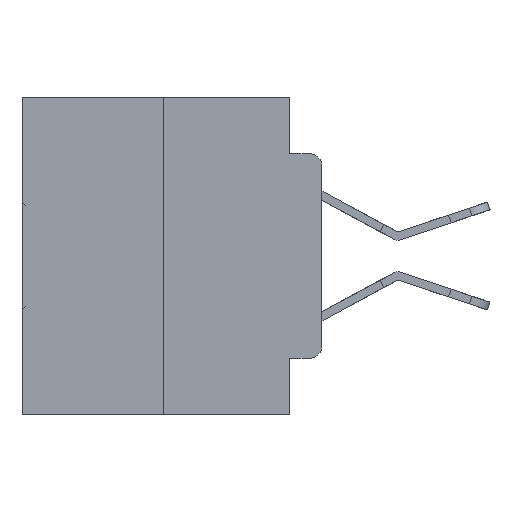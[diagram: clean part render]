
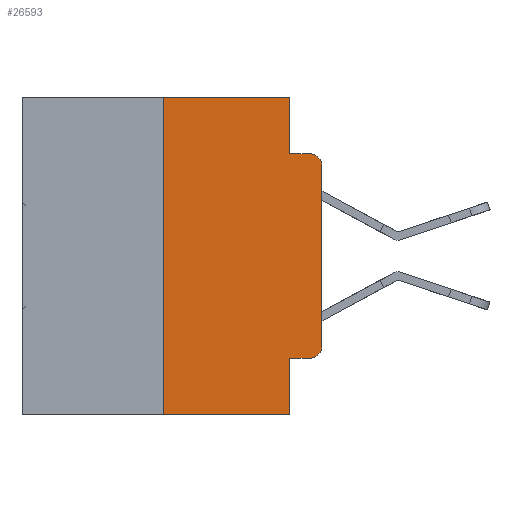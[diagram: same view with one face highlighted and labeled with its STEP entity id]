
A CAD part, left-side view. The second image highlights one B-rep face of the part: STEP entity #26593.
In plain terms, the highlighted planar face has unit normal (-1, 0, 0).
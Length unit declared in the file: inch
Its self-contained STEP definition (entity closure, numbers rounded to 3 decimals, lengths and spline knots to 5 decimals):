
#27 = CARTESIAN_POINT ( 'NONE',  ( 0., 0.051, -0.0885 ) ) ;
#431 = DIRECTION ( 'NONE',  ( 0., -1., 0. ) ) ;
#745 = CARTESIAN_POINT ( 'NONE',  ( 0., 0.051, -0.4115 ) ) ;
#867 = AXIS2_PLACEMENT_3D ( 'NONE', #20750, #5692, #33012 ) ;
#901 = LINE ( 'NONE', #29747, #17784 ) ;
#994 = VERTEX_POINT ( 'NONE', #6682 ) ;
#1021 = EDGE_CURVE ( 'NONE', #27551, #27570, #901, .T. ) ;
#2595 = LINE ( 'NONE', #27, #9815 ) ;
#2596 = ORIENTED_EDGE ( 'NONE', *, *, #13693, .T. ) ;
#2701 = ORIENTED_EDGE ( 'NONE', *, *, #3934, .T. ) ;
#2768 = VERTEX_POINT ( 'NONE', #18240 ) ;
#2932 = ORIENTED_EDGE ( 'NONE', *, *, #31230, .F. ) ;
#2973 = DIRECTION ( 'NONE',  ( 0., -1., 0. ) ) ;
#3149 = FACE_OUTER_BOUND ( 'NONE', #29541, .T. ) ;
#3934 = EDGE_CURVE ( 'NONE', #27551, #26898, #23631, .T. ) ;
#4164 = CARTESIAN_POINT ( 'NONE',  ( 0., 0., -0.1085 ) ) ;
#5619 = CARTESIAN_POINT ( 'NONE',  ( 0., 0.25, 0. ) ) ;
#5692 = DIRECTION ( 'NONE',  ( 1., 0., 0. ) ) ;
#5788 = CARTESIAN_POINT ( 'NONE',  ( 0., 0.25, -0.5 ) ) ;
#6343 = DIRECTION ( 'NONE',  ( 0., 0., 1. ) ) ;
#6682 = CARTESIAN_POINT ( 'NONE',  ( 0., 0.02, -0.4115 ) ) ;
#7279 = VECTOR ( 'NONE', #13715, 39.37008 ) ;
#7805 = CARTESIAN_POINT ( 'NONE',  ( 0., 0., 0. ) ) ;
#8265 = LINE ( 'NONE', #26204, #10832 ) ;
#8440 = ORIENTED_EDGE ( 'NONE', *, *, #26118, .T. ) ;
#8484 = VECTOR ( 'NONE', #28814, 39.37008 ) ;
#8527 = CIRCLE ( 'NONE', #26545, 0.02 ) ;
#8709 = EDGE_CURVE ( 'NONE', #27570, #29041, #8265, .T. ) ;
#9815 = VECTOR ( 'NONE', #20842, 39.37008 ) ;
#10832 = VECTOR ( 'NONE', #431, 39.37008 ) ;
#10989 = CARTESIAN_POINT ( 'NONE',  ( 0., 0.051, 0. ) ) ;
#11209 = EDGE_CURVE ( 'NONE', #16443, #33388, #2595, .T. ) ;
#12436 = CARTESIAN_POINT ( 'NONE',  ( 0., 0.051, 0. ) ) ;
#13693 = EDGE_CURVE ( 'NONE', #16097, #994, #21564, .T. ) ;
#13715 = DIRECTION ( 'NONE',  ( 0., -1., 0. ) ) ;
#14390 = CARTESIAN_POINT ( 'NONE',  ( 0., 0.051, -0.5 ) ) ;
#14406 = CIRCLE ( 'NONE', #29677, 0.02 ) ;
#14635 = ORIENTED_EDGE ( 'NONE', *, *, #11209, .F. ) ;
#15655 = DIRECTION ( 'NONE',  ( -1., 0., 0. ) ) ;
#15794 = DIRECTION ( 'NONE',  ( 0., 0., -1. ) ) ;
#16097 = VERTEX_POINT ( 'NONE', #25193 ) ;
#16354 = CARTESIAN_POINT ( 'NONE',  ( 0., 0.051, 0. ) ) ;
#16443 = VERTEX_POINT ( 'NONE', #16570 ) ;
#16570 = CARTESIAN_POINT ( 'NONE',  ( 0., 0.051, -0.0885 ) ) ;
#17191 = DIRECTION ( 'NONE',  ( -1., 0., 0. ) ) ;
#17784 = VECTOR ( 'NONE', #6343, 39.37008 ) ;
#18180 = LINE ( 'NONE', #12436, #32018 ) ;
#18240 = CARTESIAN_POINT ( 'NONE',  ( 0., 0., -0.3915 ) ) ;
#18380 = CARTESIAN_POINT ( 'NONE',  ( 0., 0.02, -0.3915 ) ) ;
#19927 = CARTESIAN_POINT ( 'NONE',  ( 0., 0.02, -0.1085 ) ) ;
#20366 = VECTOR ( 'NONE', #15794, 39.37008 ) ;
#20750 = CARTESIAN_POINT ( 'NONE',  ( 0., 0.473, 0. ) ) ;
#20842 = DIRECTION ( 'NONE',  ( 0., -1., 0. ) ) ;
#21564 = LINE ( 'NONE', #745, #7279 ) ;
#23044 = VECTOR ( 'NONE', #2973, 39.37008 ) ;
#23481 = PLANE ( 'NONE',  #867 ) ;
#23488 = DIRECTION ( 'NONE',  ( 0., 0., -1. ) ) ;
#23491 = LINE ( 'NONE', #10989, #20366 ) ;
#23631 = LINE ( 'NONE', #28598, #23044 ) ;
#23675 = DIRECTION ( 'NONE',  ( 0., 0., -1. ) ) ;
#24698 = EDGE_CURVE ( 'NONE', #994, #2768, #14406, .T. ) ;
#25193 = CARTESIAN_POINT ( 'NONE',  ( 0., 0.051, -0.4115 ) ) ;
#25556 = ORIENTED_EDGE ( 'NONE', *, *, #1021, .F. ) ;
#26118 = EDGE_CURVE ( 'NONE', #2768, #31346, #26241, .T. ) ;
#26204 = CARTESIAN_POINT ( 'NONE',  ( 0., 0.473, 0. ) ) ;
#26241 = LINE ( 'NONE', #7805, #8484 ) ;
#26545 = AXIS2_PLACEMENT_3D ( 'NONE', #19927, #17191, #30689 ) ;
#26593 = ADVANCED_FACE ( 'NONE', ( #3149 ), #23481, .F. ) ;
#26645 = ORIENTED_EDGE ( 'NONE', *, *, #8709, .F. ) ;
#26898 = VERTEX_POINT ( 'NONE', #14390 ) ;
#27551 = VERTEX_POINT ( 'NONE', #5788 ) ;
#27570 = VERTEX_POINT ( 'NONE', #5619 ) ;
#27735 = EDGE_CURVE ( 'NONE', #29041, #16443, #18180, .T. ) ;
#27851 = ORIENTED_EDGE ( 'NONE', *, *, #27735, .F. ) ;
#28168 = CARTESIAN_POINT ( 'NONE',  ( 0., 0.02, -0.0885 ) ) ;
#28302 = ORIENTED_EDGE ( 'NONE', *, *, #28743, .T. ) ;
#28598 = CARTESIAN_POINT ( 'NONE',  ( 0., 0.473, -0.5 ) ) ;
#28743 = EDGE_CURVE ( 'NONE', #31346, #33388, #8527, .T. ) ;
#28814 = DIRECTION ( 'NONE',  ( 0., 0., 1. ) ) ;
#28979 = ORIENTED_EDGE ( 'NONE', *, *, #24698, .T. ) ;
#29041 = VERTEX_POINT ( 'NONE', #16354 ) ;
#29541 = EDGE_LOOP ( 'NONE', ( #8440, #28302, #14635, #27851, #26645, #25556, #2701, #2932, #2596, #28979 ) ) ;
#29677 = AXIS2_PLACEMENT_3D ( 'NONE', #18380, #15655, #23675 ) ;
#29747 = CARTESIAN_POINT ( 'NONE',  ( 0., 0.25, 0. ) ) ;
#30689 = DIRECTION ( 'NONE',  ( 0., 0., -1. ) ) ;
#31230 = EDGE_CURVE ( 'NONE', #16097, #26898, #23491, .T. ) ;
#31346 = VERTEX_POINT ( 'NONE', #4164 ) ;
#32018 = VECTOR ( 'NONE', #23488, 39.37008 ) ;
#33012 = DIRECTION ( 'NONE',  ( 0., 0., -1. ) ) ;
#33388 = VERTEX_POINT ( 'NONE', #28168 ) ;
